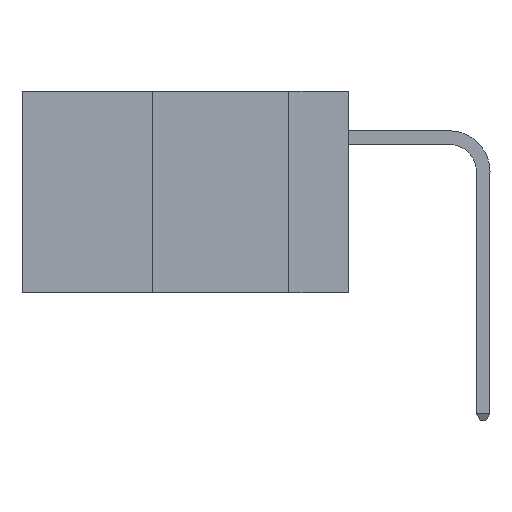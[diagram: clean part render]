
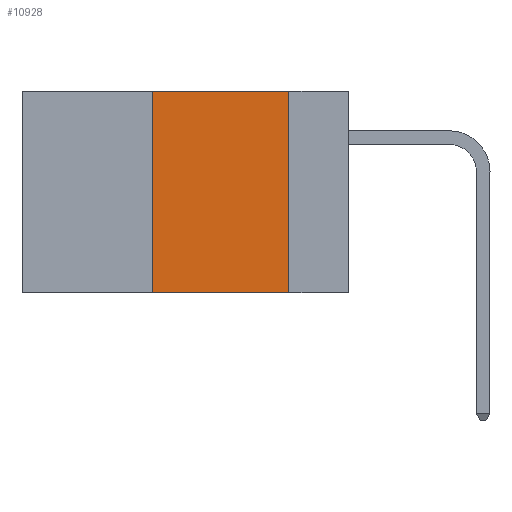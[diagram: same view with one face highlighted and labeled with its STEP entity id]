
A CAD part, left-side view. The second image highlights one B-rep face of the part: STEP entity #10928.
In plain terms, the highlighted planar face has unit normal (-1, 0, 0).
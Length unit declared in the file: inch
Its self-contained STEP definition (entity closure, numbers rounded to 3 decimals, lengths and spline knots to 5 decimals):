
#1192 = DIRECTION ( 'NONE',  ( 0., 0., -1. ) ) ;
#1314 = ORIENTED_EDGE ( 'NONE', *, *, #6327, .F. ) ;
#1378 = EDGE_LOOP ( 'NONE', ( #9967, #1314, #3895, #4259 ) ) ;
#2325 = VECTOR ( 'NONE', #10564, 39.37008 ) ;
#3231 = VECTOR ( 'NONE', #12815, 39.37008 ) ;
#3895 = ORIENTED_EDGE ( 'NONE', *, *, #6840, .F. ) ;
#4074 = CARTESIAN_POINT ( 'NONE',  ( 0., 0.11, -0.37 ) ) ;
#4259 = ORIENTED_EDGE ( 'NONE', *, *, #7432, .T. ) ;
#4575 = CARTESIAN_POINT ( 'NONE',  ( 0., 0.11, 0. ) ) ;
#4687 = CARTESIAN_POINT ( 'NONE',  ( 0., 0.6, 0. ) ) ;
#4964 = DIRECTION ( 'NONE',  ( 0., -1., 0. ) ) ;
#6208 = AXIS2_PLACEMENT_3D ( 'NONE', #4687, #8255, #1192 ) ;
#6289 = VERTEX_POINT ( 'NONE', #8430 ) ;
#6327 = EDGE_CURVE ( 'NONE', #6289, #10001, #6624, .T. ) ;
#6410 = LINE ( 'NONE', #15071, #3231 ) ;
#6624 = LINE ( 'NONE', #11973, #10837 ) ;
#6840 = EDGE_CURVE ( 'NONE', #14835, #6289, #15074, .T. ) ;
#7153 = VECTOR ( 'NONE', #8746, 39.37008 ) ;
#7432 = EDGE_CURVE ( 'NONE', #14835, #9683, #6410, .T. ) ;
#7489 = CARTESIAN_POINT ( 'NONE',  ( 0., 0.36, -0.37 ) ) ;
#8255 = DIRECTION ( 'NONE',  ( 1., 0., 0. ) ) ;
#8430 = CARTESIAN_POINT ( 'NONE',  ( 0., 0.36, 0. ) ) ;
#8746 = DIRECTION ( 'NONE',  ( 0., 0., -1. ) ) ;
#9395 = PLANE ( 'NONE',  #6208 ) ;
#9683 = VERTEX_POINT ( 'NONE', #4074 ) ;
#9967 = ORIENTED_EDGE ( 'NONE', *, *, #12320, .F. ) ;
#10001 = VERTEX_POINT ( 'NONE', #4575 ) ;
#10270 = LINE ( 'NONE', #11030, #7153 ) ;
#10514 = CARTESIAN_POINT ( 'NONE',  ( 0., 0.36, 0. ) ) ;
#10564 = DIRECTION ( 'NONE',  ( 0., 0., 1. ) ) ;
#10837 = VECTOR ( 'NONE', #4964, 39.37008 ) ;
#10928 = ADVANCED_FACE ( 'NONE', ( #12058 ), #9395, .F. ) ;
#11030 = CARTESIAN_POINT ( 'NONE',  ( 0., 0.11, 0. ) ) ;
#11973 = CARTESIAN_POINT ( 'NONE',  ( 0., 0.6, 0. ) ) ;
#12058 = FACE_OUTER_BOUND ( 'NONE', #1378, .T. ) ;
#12320 = EDGE_CURVE ( 'NONE', #10001, #9683, #10270, .T. ) ;
#12815 = DIRECTION ( 'NONE',  ( 0., -1., 0. ) ) ;
#14835 = VERTEX_POINT ( 'NONE', #7489 ) ;
#15071 = CARTESIAN_POINT ( 'NONE',  ( 0., 0.6, -0.37 ) ) ;
#15074 = LINE ( 'NONE', #10514, #2325 ) ;
